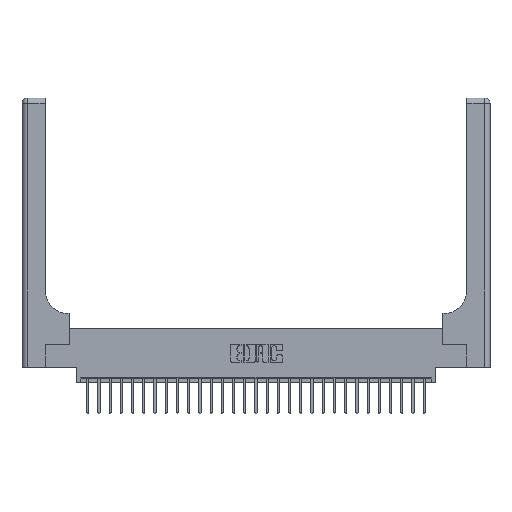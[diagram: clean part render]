
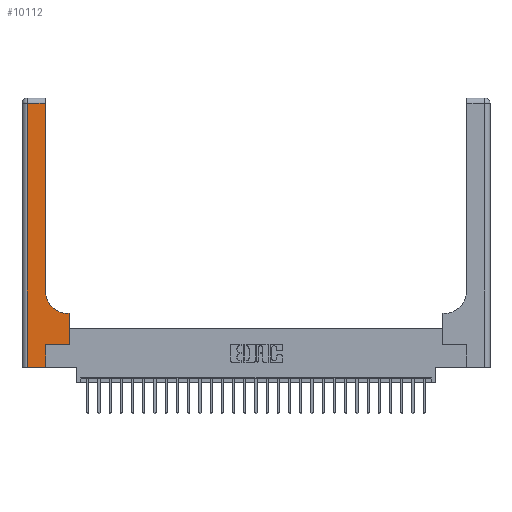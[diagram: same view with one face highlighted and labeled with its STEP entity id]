
A CAD part, top view. The second image highlights one B-rep face of the part: STEP entity #10112.
In plain terms, the highlighted planar face has unit normal (0, 0, 1).
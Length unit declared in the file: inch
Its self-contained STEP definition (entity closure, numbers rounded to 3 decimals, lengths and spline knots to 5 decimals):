
#254 = VERTEX_POINT ( 'NONE', #9764 ) ;
#402 = VERTEX_POINT ( 'NONE', #13481 ) ;
#1236 = LINE ( 'NONE', #22373, #15854 ) ;
#1494 = ORIENTED_EDGE ( 'NONE', *, *, #15354, .T. ) ;
#1770 = CIRCLE ( 'NONE', #17323, 0.25 ) ;
#2165 = EDGE_CURVE ( 'NONE', #20668, #402, #1236, .T. ) ;
#2643 = CARTESIAN_POINT ( 'NONE',  ( 0.528, 0.25, 0.37 ) ) ;
#3031 = DIRECTION ( 'NONE',  ( -1., 0., 0. ) ) ;
#3173 = FACE_OUTER_BOUND ( 'NONE', #26853, .T. ) ;
#3893 = ORIENTED_EDGE ( 'NONE', *, *, #26224, .T. ) ;
#3937 = ORIENTED_EDGE ( 'NONE', *, *, #8000, .T. ) ;
#3955 = CARTESIAN_POINT ( 'NONE',  ( 0., 0., 0.37 ) ) ;
#6116 = DIRECTION ( 'NONE',  ( 0., 0., -1. ) ) ;
#6124 = EDGE_CURVE ( 'NONE', #18958, #14942, #12799, .T. ) ;
#6332 = EDGE_CURVE ( 'NONE', #254, #20668, #1770, .T. ) ;
#6522 = DIRECTION ( 'NONE',  ( 0., 1., 0. ) ) ;
#6677 = CARTESIAN_POINT ( 'NONE',  ( 0., 2.94, 0.37 ) ) ;
#6715 = CARTESIAN_POINT ( 'NONE',  ( 0.06, 3., 0.37 ) ) ;
#6955 = LINE ( 'NONE', #6677, #8604 ) ;
#7633 = ORIENTED_EDGE ( 'NONE', *, *, #6332, .T. ) ;
#8000 = EDGE_CURVE ( 'NONE', #14942, #254, #26413, .T. ) ;
#8281 = LINE ( 'NONE', #3955, #13341 ) ;
#8385 = DIRECTION ( 'NONE',  ( 0., -1., 0. ) ) ;
#8604 = VECTOR ( 'NONE', #19322, 39.37008 ) ;
#8809 = VECTOR ( 'NONE', #6522, 39.37008 ) ;
#9480 = CARTESIAN_POINT ( 'NONE',  ( 0.528, 0.6, 0.37 ) ) ;
#9764 = CARTESIAN_POINT ( 'NONE',  ( 0.51, 0.6, 0.37 ) ) ;
#10112 = ADVANCED_FACE ( 'NONE', ( #3173 ), #26837, .F. ) ;
#12799 = LINE ( 'NONE', #2643, #24443 ) ;
#12978 = VECTOR ( 'NONE', #24325, 39.37008 ) ;
#13315 = ORIENTED_EDGE ( 'NONE', *, *, #21747, .T. ) ;
#13341 = VECTOR ( 'NONE', #18699, 39.37008 ) ;
#13469 = LINE ( 'NONE', #19465, #18783 ) ;
#13481 = CARTESIAN_POINT ( 'NONE',  ( 0.26, 2.94, 0.37 ) ) ;
#13691 = ORIENTED_EDGE ( 'NONE', *, *, #16905, .T. ) ;
#13823 = ORIENTED_EDGE ( 'NONE', *, *, #6124, .T. ) ;
#14442 = CARTESIAN_POINT ( 'NONE',  ( 0.265, 0.25, 0.37 ) ) ;
#14887 = ORIENTED_EDGE ( 'NONE', *, *, #2165, .T. ) ;
#14942 = VERTEX_POINT ( 'NONE', #9480 ) ;
#15354 = EDGE_CURVE ( 'NONE', #20898, #18958, #13469, .T. ) ;
#15854 = VECTOR ( 'NONE', #24625, 39.37008 ) ;
#15933 = VERTEX_POINT ( 'NONE', #16231 ) ;
#16231 = CARTESIAN_POINT ( 'NONE',  ( 0.06, 0., 0.37 ) ) ;
#16676 = LINE ( 'NONE', #18757, #8809 ) ;
#16905 = EDGE_CURVE ( 'NONE', #19268, #20898, #16676, .T. ) ;
#16954 = CARTESIAN_POINT ( 'NONE',  ( 0.06, 2.94, 0.37 ) ) ;
#16984 = CARTESIAN_POINT ( 'NONE',  ( 0.528, 0.25, 0.37 ) ) ;
#17323 = AXIS2_PLACEMENT_3D ( 'NONE', #20446, #6116, #26722 ) ;
#18551 = CARTESIAN_POINT ( 'NONE',  ( 0.26, 0.85, 0.37 ) ) ;
#18699 = DIRECTION ( 'NONE',  ( 1., 0., 0. ) ) ;
#18757 = CARTESIAN_POINT ( 'NONE',  ( 0.265, 0., 0.37 ) ) ;
#18783 = VECTOR ( 'NONE', #25879, 39.37008 ) ;
#18906 = ORIENTED_EDGE ( 'NONE', *, *, #23019, .T. ) ;
#18949 = LINE ( 'NONE', #6715, #23739 ) ;
#18958 = VERTEX_POINT ( 'NONE', #16984 ) ;
#19268 = VERTEX_POINT ( 'NONE', #25069 ) ;
#19288 = VERTEX_POINT ( 'NONE', #16954 ) ;
#19322 = DIRECTION ( 'NONE',  ( -1., 0., 0. ) ) ;
#19465 = CARTESIAN_POINT ( 'NONE',  ( 0.265, 0.25, 0.37 ) ) ;
#19999 = CARTESIAN_POINT ( 'NONE',  ( 0., 3., 0.37 ) ) ;
#20446 = CARTESIAN_POINT ( 'NONE',  ( 0.51, 0.85, 0.37 ) ) ;
#20668 = VERTEX_POINT ( 'NONE', #18551 ) ;
#20898 = VERTEX_POINT ( 'NONE', #14442 ) ;
#21747 = EDGE_CURVE ( 'NONE', #402, #19288, #6955, .T. ) ;
#22373 = CARTESIAN_POINT ( 'NONE',  ( 0.26, 3., 0.37 ) ) ;
#23019 = EDGE_CURVE ( 'NONE', #19288, #15933, #18949, .T. ) ;
#23526 = DIRECTION ( 'NONE',  ( 0., 1., 0. ) ) ;
#23739 = VECTOR ( 'NONE', #8385, 39.37008 ) ;
#24048 = CARTESIAN_POINT ( 'NONE',  ( 0.26, 0.6, 0.37 ) ) ;
#24325 = DIRECTION ( 'NONE',  ( -1., 0., 0. ) ) ;
#24443 = VECTOR ( 'NONE', #23526, 39.37008 ) ;
#24625 = DIRECTION ( 'NONE',  ( 0., 1., 0. ) ) ;
#25069 = CARTESIAN_POINT ( 'NONE',  ( 0.265, 0., 0.37 ) ) ;
#25879 = DIRECTION ( 'NONE',  ( 1., 0., 0. ) ) ;
#26224 = EDGE_CURVE ( 'NONE', #15933, #19268, #8281, .T. ) ;
#26413 = LINE ( 'NONE', #24048, #12978 ) ;
#26559 = DIRECTION ( 'NONE',  ( 0., 0., -1. ) ) ;
#26722 = DIRECTION ( 'NONE',  ( 1., 0., 0. ) ) ;
#26822 = AXIS2_PLACEMENT_3D ( 'NONE', #19999, #26559, #3031 ) ;
#26837 = PLANE ( 'NONE',  #26822 ) ;
#26853 = EDGE_LOOP ( 'NONE', ( #14887, #13315, #18906, #3893, #13691, #1494, #13823, #3937, #7633 ) ) ;
